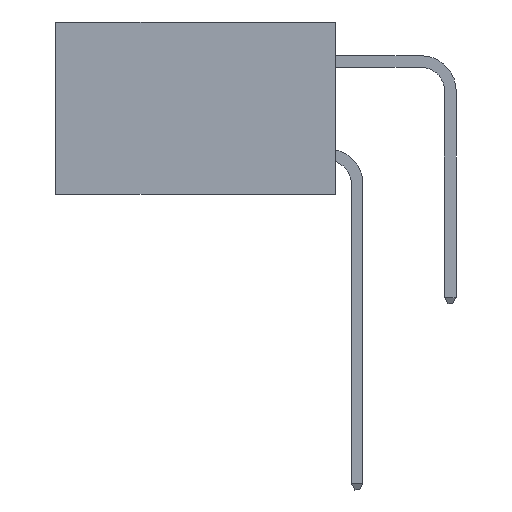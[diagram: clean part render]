
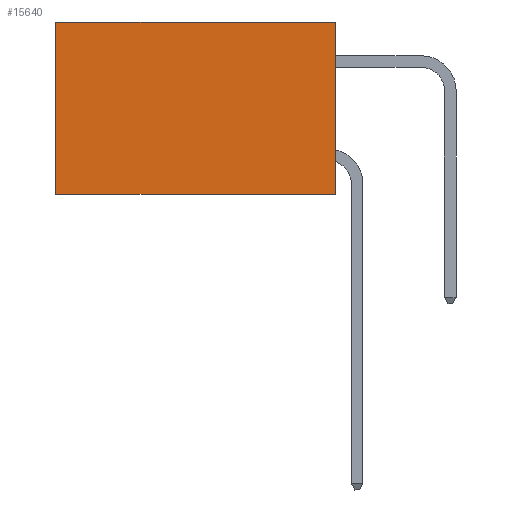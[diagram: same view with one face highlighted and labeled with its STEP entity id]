
A CAD part, left-side view. The second image highlights one B-rep face of the part: STEP entity #15640.
In plain terms, the highlighted planar face has unit normal (-1, 0, 0).
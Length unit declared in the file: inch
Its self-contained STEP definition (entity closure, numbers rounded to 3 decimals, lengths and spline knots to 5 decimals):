
#587 = CARTESIAN_POINT ( 'NONE',  ( 0.2875, 0., 0. ) ) ;
#1344 = EDGE_CURVE ( 'NONE', #21258, #22443, #16055, .T. ) ;
#3588 = LINE ( 'NONE', #28327, #11476 ) ;
#4323 = CARTESIAN_POINT ( 'NONE',  ( 0.2875, 0., 0. ) ) ;
#5197 = VECTOR ( 'NONE', #36523, 39.37008 ) ;
#6081 = EDGE_CURVE ( 'NONE', #22443, #16127, #8781, .T. ) ;
#7484 = ORIENTED_EDGE ( 'NONE', *, *, #12242, .T. ) ;
#7510 = DIRECTION ( 'NONE',  ( 1., 0., 0. ) ) ;
#8781 = LINE ( 'NONE', #24344, #27584 ) ;
#11476 = VECTOR ( 'NONE', #34614, 39.37008 ) ;
#11702 = FACE_OUTER_BOUND ( 'NONE', #29165, .T. ) ;
#12242 = EDGE_CURVE ( 'NONE', #21258, #32579, #3588, .T. ) ;
#14016 = ORIENTED_EDGE ( 'NONE', *, *, #1344, .F. ) ;
#14917 = VECTOR ( 'NONE', #23997, 39.37008 ) ;
#15640 = ADVANCED_FACE ( 'NONE', ( #11702 ), #23369, .F. ) ;
#16034 = CARTESIAN_POINT ( 'NONE',  ( 0.2875, 0.6, -0.37 ) ) ;
#16055 = LINE ( 'NONE', #30456, #5197 ) ;
#16127 = VERTEX_POINT ( 'NONE', #16034 ) ;
#16376 = LINE ( 'NONE', #32248, #14917 ) ;
#21258 = VERTEX_POINT ( 'NONE', #587 ) ;
#22443 = VERTEX_POINT ( 'NONE', #29782 ) ;
#23369 = PLANE ( 'NONE',  #37148 ) ;
#23997 = DIRECTION ( 'NONE',  ( 0., 0., -1. ) ) ;
#24344 = CARTESIAN_POINT ( 'NONE',  ( 0.2875, 0., -0.37 ) ) ;
#24823 = ORIENTED_EDGE ( 'NONE', *, *, #34353, .T. ) ;
#27460 = CARTESIAN_POINT ( 'NONE',  ( 0.2875, 0.6, 0. ) ) ;
#27584 = VECTOR ( 'NONE', #37556, 39.37008 ) ;
#28327 = CARTESIAN_POINT ( 'NONE',  ( 0.2875, 0., 0. ) ) ;
#29165 = EDGE_LOOP ( 'NONE', ( #24823, #31313, #14016, #7484 ) ) ;
#29782 = CARTESIAN_POINT ( 'NONE',  ( 0.2875, 0., -0.37 ) ) ;
#30456 = CARTESIAN_POINT ( 'NONE',  ( 0.2875, 0., 0. ) ) ;
#31313 = ORIENTED_EDGE ( 'NONE', *, *, #6081, .F. ) ;
#32248 = CARTESIAN_POINT ( 'NONE',  ( 0.2875, 0.6, 0. ) ) ;
#32579 = VERTEX_POINT ( 'NONE', #27460 ) ;
#32837 = DIRECTION ( 'NONE',  ( 0., 0., -1. ) ) ;
#34353 = EDGE_CURVE ( 'NONE', #32579, #16127, #16376, .T. ) ;
#34614 = DIRECTION ( 'NONE',  ( 0., 1., 0. ) ) ;
#36523 = DIRECTION ( 'NONE',  ( 0., 0., -1. ) ) ;
#37148 = AXIS2_PLACEMENT_3D ( 'NONE', #4323, #7510, #32837 ) ;
#37556 = DIRECTION ( 'NONE',  ( 0., 1., 0. ) ) ;
